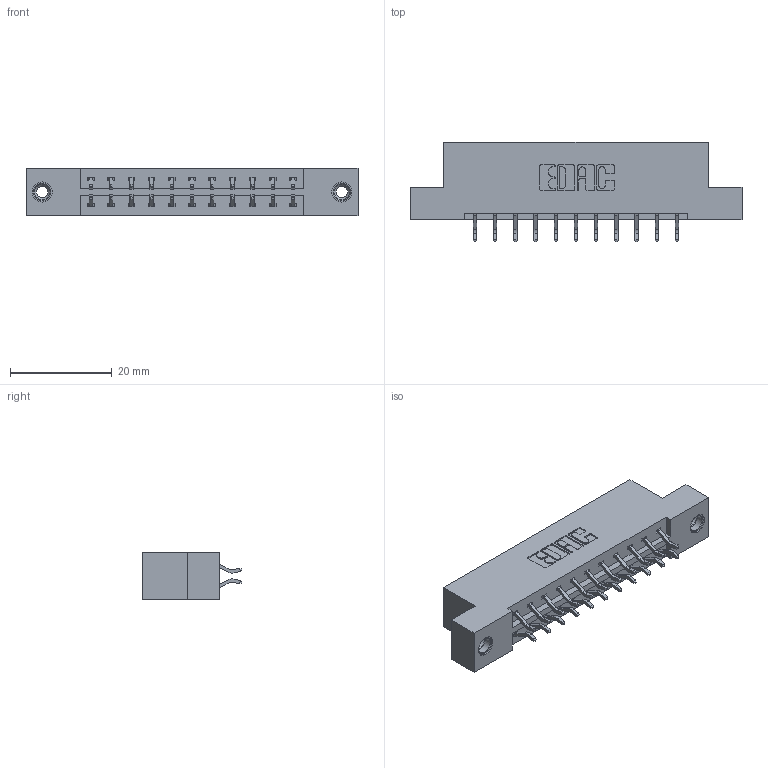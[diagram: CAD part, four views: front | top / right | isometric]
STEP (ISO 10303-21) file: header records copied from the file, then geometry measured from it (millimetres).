
FILE_DESCRIPTION (( 'STEP AP203' ), '1' );
FILE_NAME ('833-022-556-208.STEP', '2020-06-01T17:53:25', ( '' ), ( '' ), 'SwSTEP 2.0', 'SolidWorks 2020', '' );
FILE_SCHEMA (( 'CONFIG_CONTROL_DESIGN' ));
Length unit declared in the file: inch
Products named in the file (4): 345-292-001_556 Tail; 345-250-001_345-250-003-102; 833 Part_Flush - .156 Dia - TI; 833-022-556-208
Assembly tree (25 placements, depth 2):
  833-022-556-208
    833 Part_Flush - .156 Dia - TI
    345-292-001_556 Tail  x22
    345-250-001_345-250-003-102  x2
Bounding box: 65.13 x 19.57 x 9.4 mm (x, y, z)
Volume: 6351.7 mm3; surface area: 7176.2 mm2
Topology: 25 solids, 25 shells, 1450 faces, 4253 edges, 2798 vertices
Faces by surface type: plane 982, cylinder 452, cone 12, torus 4
Entity records: 12492 total; most frequent: CARTESIAN_POINT 2105, ORIENTED_EDGE 2022, DIRECTION 1873, EDGE_CURVE 1011, LINE 855, VECTOR 855, VERTEX_POINT 668, AXIS2_PLACEMENT_3D 509
